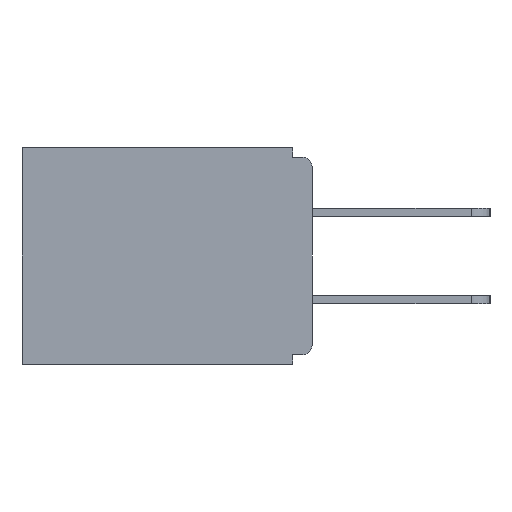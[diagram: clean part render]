
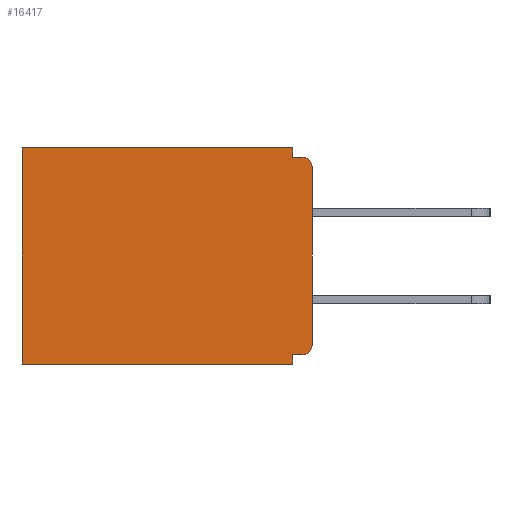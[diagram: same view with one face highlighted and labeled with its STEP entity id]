
A CAD part, left-side view. The second image highlights one B-rep face of the part: STEP entity #16417.
In plain terms, the highlighted planar face has unit normal (-1, 0, 0).
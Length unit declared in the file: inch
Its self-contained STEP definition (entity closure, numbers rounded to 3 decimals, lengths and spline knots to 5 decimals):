
#753 = LINE ( 'NONE', #13297, #18668 ) ;
#1000 = ORIENTED_EDGE ( 'NONE', *, *, #11362, .F. ) ;
#1048 = VECTOR ( 'NONE', #19404, 39.37008 ) ;
#1310 = LINE ( 'NONE', #1669, #1048 ) ;
#1669 = CARTESIAN_POINT ( 'NONE',  ( 0.298, 0., -0.015 ) ) ;
#2754 = VERTEX_POINT ( 'NONE', #5615 ) ;
#2960 = CARTESIAN_POINT ( 'NONE',  ( 0.298, 0.015, -0.015 ) ) ;
#3101 = VERTEX_POINT ( 'NONE', #16805 ) ;
#3238 = ORIENTED_EDGE ( 'NONE', *, *, #5927, .F. ) ;
#3604 = EDGE_LOOP ( 'NONE', ( #17447, #5100, #1000, #13243, #14472, #3238, #17816, #13129, #4897, #13833 ) ) ;
#3985 = AXIS2_PLACEMENT_3D ( 'NONE', #18568, #10311, #13709 ) ;
#4897 = ORIENTED_EDGE ( 'NONE', *, *, #16206, .T. ) ;
#4982 = VECTOR ( 'NONE', #12314, 39.37008 ) ;
#5100 = ORIENTED_EDGE ( 'NONE', *, *, #5334, .F. ) ;
#5334 = EDGE_CURVE ( 'NONE', #13025, #21000, #1310, .T. ) ;
#5523 = AXIS2_PLACEMENT_3D ( 'NONE', #11429, #18233, #18020 ) ;
#5615 = CARTESIAN_POINT ( 'NONE',  ( 0.298, 0.015, -0.328 ) ) ;
#5927 = EDGE_CURVE ( 'NONE', #18704, #3101, #9742, .T. ) ;
#6219 = DIRECTION ( 'NONE',  ( 0., 1., 0. ) ) ;
#6487 = EDGE_CURVE ( 'NONE', #10299, #21000, #15076, .T. ) ;
#6550 = EDGE_CURVE ( 'NONE', #16353, #18704, #16079, .T. ) ;
#6653 = DIRECTION ( 'NONE',  ( 0., 0., -1. ) ) ;
#7230 = CARTESIAN_POINT ( 'NONE',  ( 0.298, 0.46, 0. ) ) ;
#7334 = CARTESIAN_POINT ( 'NONE',  ( 0.298, 0.031, -0.015 ) ) ;
#8998 = CIRCLE ( 'NONE', #12910, 0.015 ) ;
#9229 = VECTOR ( 'NONE', #21042, 39.37008 ) ;
#9482 = DIRECTION ( 'NONE',  ( -1., 0., 0. ) ) ;
#9742 = LINE ( 'NONE', #15981, #18183 ) ;
#9827 = DIRECTION ( 'NONE',  ( 0., 0., -1. ) ) ;
#10000 = VECTOR ( 'NONE', #6653, 39.37008 ) ;
#10186 = CARTESIAN_POINT ( 'NONE',  ( 0.298, 0., 0. ) ) ;
#10263 = DIRECTION ( 'NONE',  ( 0., 1., 0. ) ) ;
#10299 = VERTEX_POINT ( 'NONE', #20154 ) ;
#10311 = DIRECTION ( 'NONE',  ( -1., 0., 0. ) ) ;
#10328 = VERTEX_POINT ( 'NONE', #7230 ) ;
#10774 = EDGE_CURVE ( 'NONE', #10328, #3101, #12549, .T. ) ;
#11019 = LINE ( 'NONE', #10186, #10000 ) ;
#11039 = DIRECTION ( 'NONE',  ( 0., 0., -1. ) ) ;
#11362 = EDGE_CURVE ( 'NONE', #17204, #13025, #753, .T. ) ;
#11429 = CARTESIAN_POINT ( 'NONE',  ( 0.298, 0., 0. ) ) ;
#12306 = CARTESIAN_POINT ( 'NONE',  ( 0.298, 0.031, -0.343 ) ) ;
#12314 = DIRECTION ( 'NONE',  ( 0., 1., 0. ) ) ;
#12549 = LINE ( 'NONE', #17820, #9229 ) ;
#12910 = AXIS2_PLACEMENT_3D ( 'NONE', #20850, #9482, #11039 ) ;
#13025 = VERTEX_POINT ( 'NONE', #7334 ) ;
#13129 = ORIENTED_EDGE ( 'NONE', *, *, #18595, .F. ) ;
#13243 = ORIENTED_EDGE ( 'NONE', *, *, #15299, .T. ) ;
#13297 = CARTESIAN_POINT ( 'NONE',  ( 0.298, 0.031, -0.343 ) ) ;
#13547 = VECTOR ( 'NONE', #13861, 39.37008 ) ;
#13681 = LINE ( 'NONE', #18814, #4982 ) ;
#13709 = DIRECTION ( 'NONE',  ( 0., 0., -1. ) ) ;
#13833 = ORIENTED_EDGE ( 'NONE', *, *, #17498, .F. ) ;
#13861 = DIRECTION ( 'NONE',  ( 0., 0., -1. ) ) ;
#14472 = ORIENTED_EDGE ( 'NONE', *, *, #10774, .T. ) ;
#15076 = CIRCLE ( 'NONE', #3985, 0.015 ) ;
#15299 = EDGE_CURVE ( 'NONE', #17204, #10328, #13681, .T. ) ;
#15981 = CARTESIAN_POINT ( 'NONE',  ( 0.298, 0., -0.343 ) ) ;
#16079 = LINE ( 'NONE', #18843, #13547 ) ;
#16084 = LINE ( 'NONE', #16929, #17365 ) ;
#16206 = EDGE_CURVE ( 'NONE', #2754, #20949, #8998, .T. ) ;
#16353 = VERTEX_POINT ( 'NONE', #19797 ) ;
#16417 = ADVANCED_FACE ( 'NONE', ( #19484 ), #18301, .F. ) ;
#16805 = CARTESIAN_POINT ( 'NONE',  ( 0.298, 0.46, -0.343 ) ) ;
#16929 = CARTESIAN_POINT ( 'NONE',  ( 0.298, 0., -0.328 ) ) ;
#17204 = VERTEX_POINT ( 'NONE', #20414 ) ;
#17365 = VECTOR ( 'NONE', #10263, 39.37008 ) ;
#17447 = ORIENTED_EDGE ( 'NONE', *, *, #6487, .T. ) ;
#17498 = EDGE_CURVE ( 'NONE', #10299, #20949, #11019, .T. ) ;
#17621 = CARTESIAN_POINT ( 'NONE',  ( 0.298, 0., -0.313 ) ) ;
#17816 = ORIENTED_EDGE ( 'NONE', *, *, #6550, .F. ) ;
#17820 = CARTESIAN_POINT ( 'NONE',  ( 0.298, 0.46, 0. ) ) ;
#18020 = DIRECTION ( 'NONE',  ( 0., 0., -1. ) ) ;
#18183 = VECTOR ( 'NONE', #6219, 39.37008 ) ;
#18233 = DIRECTION ( 'NONE',  ( 1., 0., 0. ) ) ;
#18301 = PLANE ( 'NONE',  #5523 ) ;
#18568 = CARTESIAN_POINT ( 'NONE',  ( 0.298, 0.015, -0.03 ) ) ;
#18595 = EDGE_CURVE ( 'NONE', #2754, #16353, #16084, .T. ) ;
#18668 = VECTOR ( 'NONE', #9827, 39.37008 ) ;
#18704 = VERTEX_POINT ( 'NONE', #12306 ) ;
#18814 = CARTESIAN_POINT ( 'NONE',  ( 0.298, 0., 0. ) ) ;
#18843 = CARTESIAN_POINT ( 'NONE',  ( 0.298, 0.031, -0.343 ) ) ;
#19404 = DIRECTION ( 'NONE',  ( 0., -1., 0. ) ) ;
#19484 = FACE_OUTER_BOUND ( 'NONE', #3604, .T. ) ;
#19797 = CARTESIAN_POINT ( 'NONE',  ( 0.298, 0.031, -0.328 ) ) ;
#20154 = CARTESIAN_POINT ( 'NONE',  ( 0.298, 0., -0.03 ) ) ;
#20414 = CARTESIAN_POINT ( 'NONE',  ( 0.298, 0.031, 0. ) ) ;
#20850 = CARTESIAN_POINT ( 'NONE',  ( 0.298, 0.015, -0.313 ) ) ;
#20949 = VERTEX_POINT ( 'NONE', #17621 ) ;
#21000 = VERTEX_POINT ( 'NONE', #2960 ) ;
#21042 = DIRECTION ( 'NONE',  ( 0., 0., -1. ) ) ;
